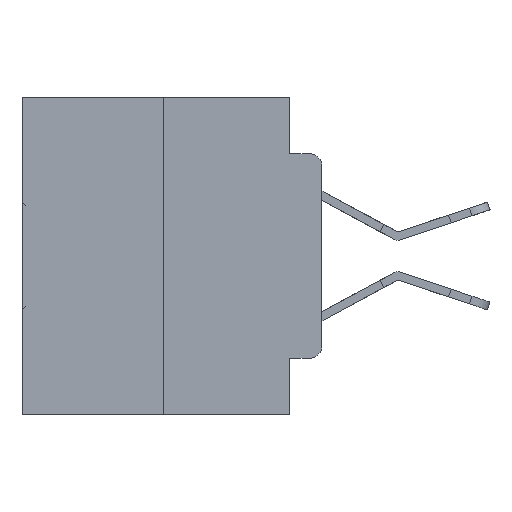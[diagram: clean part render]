
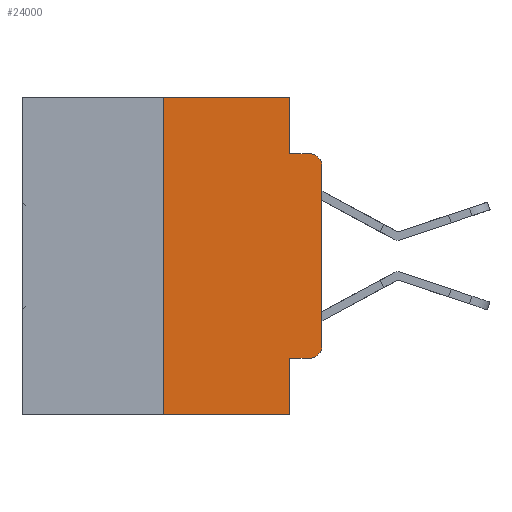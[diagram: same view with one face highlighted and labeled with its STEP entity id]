
A CAD part, left-side view. The second image highlights one B-rep face of the part: STEP entity #24000.
In plain terms, the highlighted planar face has unit normal (-1, 0, 0).
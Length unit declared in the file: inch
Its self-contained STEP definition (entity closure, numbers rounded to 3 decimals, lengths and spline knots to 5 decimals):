
#268 = DIRECTION ( 'NONE',  ( -1., 0., 0. ) ) ;
#440 = CARTESIAN_POINT ( 'NONE',  ( 0., 0.051, -0.4115 ) ) ;
#1521 = ORIENTED_EDGE ( 'NONE', *, *, #13777, .T. ) ;
#2322 = VERTEX_POINT ( 'NONE', #16594 ) ;
#2340 = LINE ( 'NONE', #17353, #17764 ) ;
#3301 = EDGE_CURVE ( 'NONE', #10950, #2322, #2340, .T. ) ;
#3558 = EDGE_CURVE ( 'NONE', #10950, #30452, #15508, .T. ) ;
#3956 = CARTESIAN_POINT ( 'NONE',  ( 0., 0.02, -0.3915 ) ) ;
#4119 = LINE ( 'NONE', #23955, #8972 ) ;
#4220 = VECTOR ( 'NONE', #7522, 39.37008 ) ;
#4731 = ORIENTED_EDGE ( 'NONE', *, *, #23599, .T. ) ;
#4851 = DIRECTION ( 'NONE',  ( 0., -1., 0. ) ) ;
#4909 = CARTESIAN_POINT ( 'NONE',  ( 0., 0.051, -0.5 ) ) ;
#5159 = ORIENTED_EDGE ( 'NONE', *, *, #9591, .T. ) ;
#5324 = ORIENTED_EDGE ( 'NONE', *, *, #17836, .F. ) ;
#5476 = VECTOR ( 'NONE', #29506, 39.37008 ) ;
#5504 = DIRECTION ( 'NONE',  ( 0., -1., 0. ) ) ;
#6412 = CARTESIAN_POINT ( 'NONE',  ( 0., 0.473, 0. ) ) ;
#6930 = PLANE ( 'NONE',  #21533 ) ;
#6962 = EDGE_CURVE ( 'NONE', #26396, #30780, #29841, .T. ) ;
#7522 = DIRECTION ( 'NONE',  ( 0., 0., -1. ) ) ;
#7746 = CARTESIAN_POINT ( 'NONE',  ( 0., 0.25, -0.5 ) ) ;
#8972 = VECTOR ( 'NONE', #16780, 39.37008 ) ;
#9359 = CARTESIAN_POINT ( 'NONE',  ( 0., 0.25, 0. ) ) ;
#9591 = EDGE_CURVE ( 'NONE', #9850, #23797, #25655, .T. ) ;
#9850 = VERTEX_POINT ( 'NONE', #30064 ) ;
#9865 = CARTESIAN_POINT ( 'NONE',  ( 0., 0.051, 0. ) ) ;
#10216 = VERTEX_POINT ( 'NONE', #26869 ) ;
#10950 = VERTEX_POINT ( 'NONE', #440 ) ;
#11255 = FACE_OUTER_BOUND ( 'NONE', #23604, .T. ) ;
#11271 = AXIS2_PLACEMENT_3D ( 'NONE', #32641, #268, #12485 ) ;
#12062 = CARTESIAN_POINT ( 'NONE',  ( 0., 0., 0. ) ) ;
#12485 = DIRECTION ( 'NONE',  ( 0., 0., -1. ) ) ;
#13018 = CARTESIAN_POINT ( 'NONE',  ( 0., 0.473, -0.5 ) ) ;
#13186 = DIRECTION ( 'NONE',  ( 0., 0., -1. ) ) ;
#13419 = ORIENTED_EDGE ( 'NONE', *, *, #3558, .F. ) ;
#13777 = EDGE_CURVE ( 'NONE', #28109, #9850, #24234, .T. ) ;
#15508 = LINE ( 'NONE', #28511, #30099 ) ;
#15597 = CARTESIAN_POINT ( 'NONE',  ( 0., 0.02, -0.0885 ) ) ;
#16560 = DIRECTION ( 'NONE',  ( 0., -1., 0. ) ) ;
#16594 = CARTESIAN_POINT ( 'NONE',  ( 0., 0.02, -0.4115 ) ) ;
#16780 = DIRECTION ( 'NONE',  ( 0., -1., 0. ) ) ;
#17353 = CARTESIAN_POINT ( 'NONE',  ( 0., 0.051, -0.4115 ) ) ;
#17764 = VECTOR ( 'NONE', #4851, 39.37008 ) ;
#17836 = EDGE_CURVE ( 'NONE', #10216, #23797, #4119, .T. ) ;
#19782 = DIRECTION ( 'NONE',  ( -1., 0., 0. ) ) ;
#20212 = VECTOR ( 'NONE', #16560, 39.37008 ) ;
#20492 = EDGE_CURVE ( 'NONE', #30780, #25903, #32560, .T. ) ;
#20701 = CARTESIAN_POINT ( 'NONE',  ( 0., 0., -0.3915 ) ) ;
#21167 = EDGE_CURVE ( 'NONE', #26396, #30452, #28339, .T. ) ;
#21533 = AXIS2_PLACEMENT_3D ( 'NONE', #29249, #29083, #27093 ) ;
#23132 = CIRCLE ( 'NONE', #25297, 0.02 ) ;
#23599 = EDGE_CURVE ( 'NONE', #2322, #28109, #23132, .T. ) ;
#23604 = EDGE_LOOP ( 'NONE', ( #1521, #5159, #5324, #29176, #26008, #31921, #28174, #13419, #27304, #4731 ) ) ;
#23797 = VERTEX_POINT ( 'NONE', #15597 ) ;
#23955 = CARTESIAN_POINT ( 'NONE',  ( 0., 0.051, -0.0885 ) ) ;
#24000 = ADVANCED_FACE ( 'NONE', ( #11255 ), #6930, .F. ) ;
#24234 = LINE ( 'NONE', #12062, #32180 ) ;
#25297 = AXIS2_PLACEMENT_3D ( 'NONE', #3956, #19782, #26626 ) ;
#25655 = CIRCLE ( 'NONE', #11271, 0.02 ) ;
#25903 = VERTEX_POINT ( 'NONE', #32536 ) ;
#26008 = ORIENTED_EDGE ( 'NONE', *, *, #20492, .F. ) ;
#26396 = VERTEX_POINT ( 'NONE', #7746 ) ;
#26626 = DIRECTION ( 'NONE',  ( 0., 0., -1. ) ) ;
#26869 = CARTESIAN_POINT ( 'NONE',  ( 0., 0.051, -0.0885 ) ) ;
#27093 = DIRECTION ( 'NONE',  ( 0., 0., -1. ) ) ;
#27304 = ORIENTED_EDGE ( 'NONE', *, *, #3301, .T. ) ;
#28109 = VERTEX_POINT ( 'NONE', #20701 ) ;
#28174 = ORIENTED_EDGE ( 'NONE', *, *, #21167, .T. ) ;
#28339 = LINE ( 'NONE', #13018, #32588 ) ;
#28511 = CARTESIAN_POINT ( 'NONE',  ( 0., 0.051, 0. ) ) ;
#29083 = DIRECTION ( 'NONE',  ( 1., 0., 0. ) ) ;
#29176 = ORIENTED_EDGE ( 'NONE', *, *, #29821, .F. ) ;
#29249 = CARTESIAN_POINT ( 'NONE',  ( 0., 0.473, 0. ) ) ;
#29506 = DIRECTION ( 'NONE',  ( 0., 0., 1. ) ) ;
#29821 = EDGE_CURVE ( 'NONE', #25903, #10216, #32686, .T. ) ;
#29841 = LINE ( 'NONE', #9359, #5476 ) ;
#30064 = CARTESIAN_POINT ( 'NONE',  ( 0., 0., -0.1085 ) ) ;
#30099 = VECTOR ( 'NONE', #13186, 39.37008 ) ;
#30452 = VERTEX_POINT ( 'NONE', #4909 ) ;
#30469 = CARTESIAN_POINT ( 'NONE',  ( 0., 0.25, 0. ) ) ;
#30780 = VERTEX_POINT ( 'NONE', #30469 ) ;
#31921 = ORIENTED_EDGE ( 'NONE', *, *, #6962, .F. ) ;
#32180 = VECTOR ( 'NONE', #32226, 39.37008 ) ;
#32226 = DIRECTION ( 'NONE',  ( 0., 0., 1. ) ) ;
#32536 = CARTESIAN_POINT ( 'NONE',  ( 0., 0.051, 0. ) ) ;
#32560 = LINE ( 'NONE', #6412, #20212 ) ;
#32588 = VECTOR ( 'NONE', #5504, 39.37008 ) ;
#32641 = CARTESIAN_POINT ( 'NONE',  ( 0., 0.02, -0.1085 ) ) ;
#32686 = LINE ( 'NONE', #9865, #4220 ) ;
